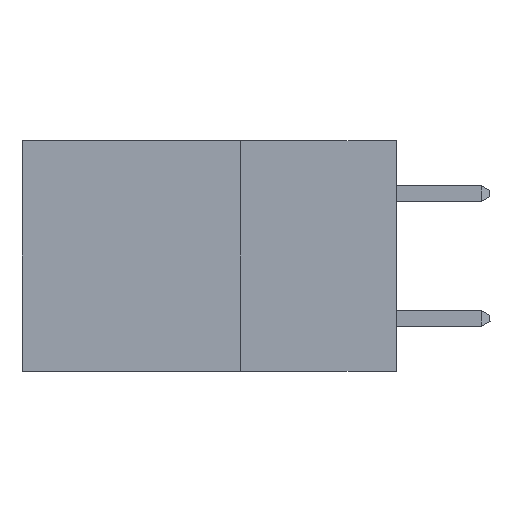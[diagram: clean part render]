
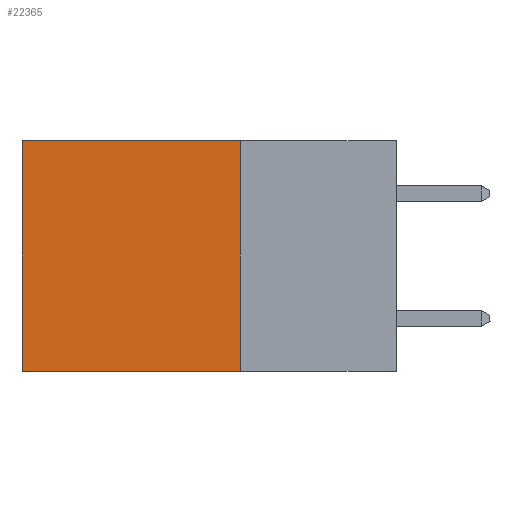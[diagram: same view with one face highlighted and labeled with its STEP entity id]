
A CAD part, left-side view. The second image highlights one B-rep face of the part: STEP entity #22365.
In plain terms, the highlighted planar face has unit normal (-1, 0, 0).
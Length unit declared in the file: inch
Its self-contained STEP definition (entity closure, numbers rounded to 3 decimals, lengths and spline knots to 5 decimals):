
#237 = DIRECTION ( 'NONE',  ( 0., 0., -1. ) ) ;
#656 = VECTOR ( 'NONE', #761, 39.37008 ) ;
#761 = DIRECTION ( 'NONE',  ( 0., 0., -1. ) ) ;
#1946 = EDGE_CURVE ( 'NONE', #24139, #16488, #15625, .T. ) ;
#2250 = ORIENTED_EDGE ( 'NONE', *, *, #1946, .F. ) ;
#3494 = VERTEX_POINT ( 'NONE', #3795 ) ;
#3666 = DIRECTION ( 'NONE',  ( 0., 1., 0. ) ) ;
#3795 = CARTESIAN_POINT ( 'NONE',  ( 0.298, 0.6, -0.37 ) ) ;
#4199 = DIRECTION ( 'NONE',  ( 1., 0., 0. ) ) ;
#6028 = VECTOR ( 'NONE', #237, 39.37008 ) ;
#7715 = EDGE_CURVE ( 'NONE', #24139, #18462, #20916, .T. ) ;
#9342 = VECTOR ( 'NONE', #27413, 39.37008 ) ;
#10399 = CARTESIAN_POINT ( 'NONE',  ( 0.298, 0.25, 0. ) ) ;
#10660 = CARTESIAN_POINT ( 'NONE',  ( 0.298, 0.25, 0. ) ) ;
#11349 = LINE ( 'NONE', #23109, #22176 ) ;
#11829 = LINE ( 'NONE', #24084, #6028 ) ;
#12761 = AXIS2_PLACEMENT_3D ( 'NONE', #10660, #4199, #19385 ) ;
#12839 = EDGE_LOOP ( 'NONE', ( #15147, #17356, #2250, #17595 ) ) ;
#13687 = CARTESIAN_POINT ( 'NONE',  ( 0.298, 0.25, -0.37 ) ) ;
#15147 = ORIENTED_EDGE ( 'NONE', *, *, #17030, .T. ) ;
#15625 = LINE ( 'NONE', #20759, #656 ) ;
#16488 = VERTEX_POINT ( 'NONE', #13687 ) ;
#17030 = EDGE_CURVE ( 'NONE', #18462, #3494, #11829, .T. ) ;
#17186 = PLANE ( 'NONE',  #12761 ) ;
#17356 = ORIENTED_EDGE ( 'NONE', *, *, #24041, .F. ) ;
#17595 = ORIENTED_EDGE ( 'NONE', *, *, #7715, .T. ) ;
#18462 = VERTEX_POINT ( 'NONE', #25198 ) ;
#18828 = CARTESIAN_POINT ( 'NONE',  ( 0.298, 0.25, 0. ) ) ;
#19385 = DIRECTION ( 'NONE',  ( 0., 0., -1. ) ) ;
#20759 = CARTESIAN_POINT ( 'NONE',  ( 0.298, 0.25, 0. ) ) ;
#20916 = LINE ( 'NONE', #18828, #9342 ) ;
#21691 = FACE_OUTER_BOUND ( 'NONE', #12839, .T. ) ;
#22176 = VECTOR ( 'NONE', #3666, 39.37008 ) ;
#22365 = ADVANCED_FACE ( 'NONE', ( #21691 ), #17186, .F. ) ;
#23109 = CARTESIAN_POINT ( 'NONE',  ( 0.298, 0.25, -0.37 ) ) ;
#24041 = EDGE_CURVE ( 'NONE', #16488, #3494, #11349, .T. ) ;
#24084 = CARTESIAN_POINT ( 'NONE',  ( 0.298, 0.6, 0. ) ) ;
#24139 = VERTEX_POINT ( 'NONE', #10399 ) ;
#25198 = CARTESIAN_POINT ( 'NONE',  ( 0.298, 0.6, 0. ) ) ;
#27413 = DIRECTION ( 'NONE',  ( 0., 1., 0. ) ) ;
